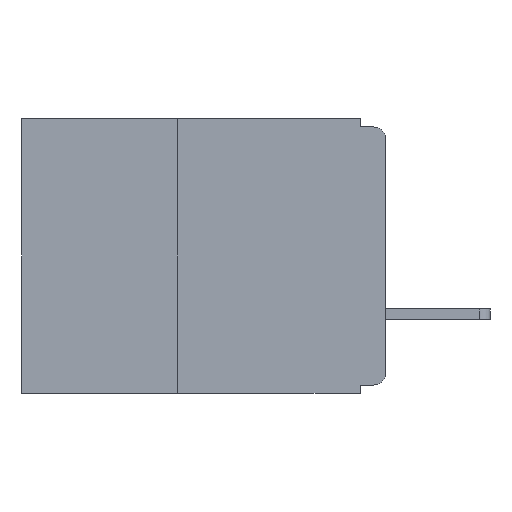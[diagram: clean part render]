
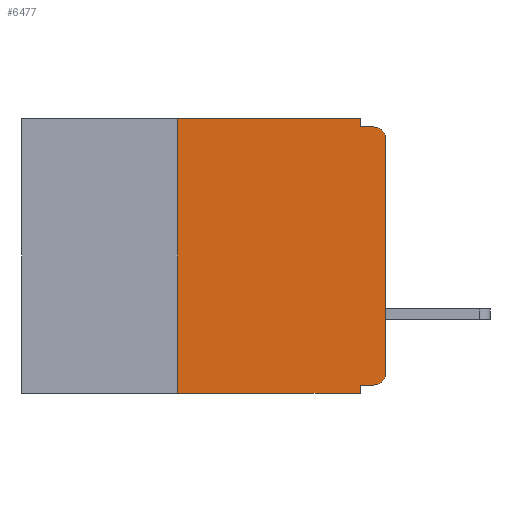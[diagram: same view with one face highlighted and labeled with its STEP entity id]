
A CAD part, left-side view. The second image highlights one B-rep face of the part: STEP entity #6477.
In plain terms, the highlighted planar face has unit normal (-1, 0, 0).
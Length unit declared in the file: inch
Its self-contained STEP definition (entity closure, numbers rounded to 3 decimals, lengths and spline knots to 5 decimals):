
#161 = ORIENTED_EDGE ( 'NONE', *, *, #11580, .F. ) ;
#552 = CARTESIAN_POINT ( 'NONE',  ( 0., 0., -0.01 ) ) ;
#624 = DIRECTION ( 'NONE',  ( 0., -1., 0. ) ) ;
#944 = VERTEX_POINT ( 'NONE', #4476 ) ;
#1103 = DIRECTION ( 'NONE',  ( -1., 0., 0. ) ) ;
#2152 = CARTESIAN_POINT ( 'NONE',  ( 0., 0.031, -0.33 ) ) ;
#2532 = EDGE_CURVE ( 'NONE', #5819, #17092, #18656, .T. ) ;
#2851 = DIRECTION ( 'NONE',  ( 0., 0., 1. ) ) ;
#3245 = VECTOR ( 'NONE', #624, 39.37008 ) ;
#3346 = CARTESIAN_POINT ( 'NONE',  ( 0., 0.25, 0. ) ) ;
#3516 = VERTEX_POINT ( 'NONE', #11714 ) ;
#3613 = LINE ( 'NONE', #552, #12341 ) ;
#3626 = ORIENTED_EDGE ( 'NONE', *, *, #19612, .T. ) ;
#3644 = CARTESIAN_POINT ( 'NONE',  ( 0., 0.031, -0.32 ) ) ;
#3839 = CARTESIAN_POINT ( 'NONE',  ( 0., 0.25, -0.33 ) ) ;
#4476 = CARTESIAN_POINT ( 'NONE',  ( 0., 0.015, -0.32 ) ) ;
#5031 = CARTESIAN_POINT ( 'NONE',  ( 0., 0.015, -0.01 ) ) ;
#5152 = ORIENTED_EDGE ( 'NONE', *, *, #12408, .T. ) ;
#5431 = CARTESIAN_POINT ( 'NONE',  ( 0., 0.031, 0. ) ) ;
#5499 = DIRECTION ( 'NONE',  ( 0., 0., -1. ) ) ;
#5501 = DIRECTION ( 'NONE',  ( 1., 0., 0. ) ) ;
#5657 = PLANE ( 'NONE',  #17679 ) ;
#5690 = LINE ( 'NONE', #8557, #14401 ) ;
#5729 = CARTESIAN_POINT ( 'NONE',  ( 0., 0.437, 0. ) ) ;
#5819 = VERTEX_POINT ( 'NONE', #21030 ) ;
#6320 = AXIS2_PLACEMENT_3D ( 'NONE', #11506, #1103, #13298 ) ;
#6477 = ADVANCED_FACE ( 'NONE', ( #7716 ), #5657, .F. ) ;
#6663 = ORIENTED_EDGE ( 'NONE', *, *, #12647, .F. ) ;
#6721 = ORIENTED_EDGE ( 'NONE', *, *, #19147, .F. ) ;
#7189 = EDGE_CURVE ( 'NONE', #19996, #3516, #12855, .T. ) ;
#7716 = FACE_OUTER_BOUND ( 'NONE', #10696, .T. ) ;
#7891 = LINE ( 'NONE', #11055, #3245 ) ;
#8170 = VERTEX_POINT ( 'NONE', #2152 ) ;
#8555 = VERTEX_POINT ( 'NONE', #5031 ) ;
#8557 = CARTESIAN_POINT ( 'NONE',  ( 0., 0., -0.32 ) ) ;
#8619 = CARTESIAN_POINT ( 'NONE',  ( 0., 0.031, -0.33 ) ) ;
#8754 = CIRCLE ( 'NONE', #19725, 0.015 ) ;
#9518 = CARTESIAN_POINT ( 'NONE',  ( 0., 0.015, -0.025 ) ) ;
#10535 = CARTESIAN_POINT ( 'NONE',  ( 0., 0.031, -0.01 ) ) ;
#10696 = EDGE_LOOP ( 'NONE', ( #18033, #5152, #161, #20203, #15067, #21837, #20244, #6663, #6721, #3626 ) ) ;
#11055 = CARTESIAN_POINT ( 'NONE',  ( 0., 0.437, -0.33 ) ) ;
#11281 = DIRECTION ( 'NONE',  ( 0., 0., -1. ) ) ;
#11506 = CARTESIAN_POINT ( 'NONE',  ( 0., 0.015, -0.305 ) ) ;
#11580 = EDGE_CURVE ( 'NONE', #13933, #8555, #3613, .T. ) ;
#11679 = DIRECTION ( 'NONE',  ( 0., 0., 1. ) ) ;
#11714 = CARTESIAN_POINT ( 'NONE',  ( 0., 0., -0.025 ) ) ;
#12341 = VECTOR ( 'NONE', #12736, 39.37008 ) ;
#12408 = EDGE_CURVE ( 'NONE', #3516, #8555, #8754, .T. ) ;
#12574 = CARTESIAN_POINT ( 'NONE',  ( 0., 0., -0.305 ) ) ;
#12647 = EDGE_CURVE ( 'NONE', #18628, #8170, #17695, .T. ) ;
#12736 = DIRECTION ( 'NONE',  ( 0., -1., 0. ) ) ;
#12855 = LINE ( 'NONE', #21897, #21871 ) ;
#13130 = VECTOR ( 'NONE', #20693, 39.37008 ) ;
#13298 = DIRECTION ( 'NONE',  ( 0., 0., -1. ) ) ;
#13933 = VERTEX_POINT ( 'NONE', #10535 ) ;
#14125 = VECTOR ( 'NONE', #2851, 39.37008 ) ;
#14271 = LINE ( 'NONE', #17498, #18278 ) ;
#14401 = VECTOR ( 'NONE', #20570, 39.37008 ) ;
#14934 = CIRCLE ( 'NONE', #6320, 0.015 ) ;
#15067 = ORIENTED_EDGE ( 'NONE', *, *, #22327, .F. ) ;
#15164 = VECTOR ( 'NONE', #21549, 39.37008 ) ;
#15699 = LINE ( 'NONE', #19882, #15164 ) ;
#17092 = VERTEX_POINT ( 'NONE', #3346 ) ;
#17199 = VERTEX_POINT ( 'NONE', #5431 ) ;
#17498 = CARTESIAN_POINT ( 'NONE',  ( 0., 0.437, 0. ) ) ;
#17679 = AXIS2_PLACEMENT_3D ( 'NONE', #5729, #5501, #5499 ) ;
#17695 = LINE ( 'NONE', #8619, #13130 ) ;
#18033 = ORIENTED_EDGE ( 'NONE', *, *, #7189, .T. ) ;
#18246 = EDGE_CURVE ( 'NONE', #5819, #8170, #7891, .T. ) ;
#18278 = VECTOR ( 'NONE', #19166, 39.37008 ) ;
#18628 = VERTEX_POINT ( 'NONE', #3644 ) ;
#18656 = LINE ( 'NONE', #3839, #14125 ) ;
#19147 = EDGE_CURVE ( 'NONE', #944, #18628, #5690, .T. ) ;
#19166 = DIRECTION ( 'NONE',  ( 0., -1., 0. ) ) ;
#19612 = EDGE_CURVE ( 'NONE', #944, #19996, #14934, .T. ) ;
#19725 = AXIS2_PLACEMENT_3D ( 'NONE', #9518, #21494, #11281 ) ;
#19882 = CARTESIAN_POINT ( 'NONE',  ( 0., 0.031, 0. ) ) ;
#19996 = VERTEX_POINT ( 'NONE', #12574 ) ;
#20154 = EDGE_CURVE ( 'NONE', #17199, #13933, #15699, .T. ) ;
#20203 = ORIENTED_EDGE ( 'NONE', *, *, #20154, .F. ) ;
#20244 = ORIENTED_EDGE ( 'NONE', *, *, #18246, .T. ) ;
#20570 = DIRECTION ( 'NONE',  ( 0., 1., 0. ) ) ;
#20693 = DIRECTION ( 'NONE',  ( 0., 0., -1. ) ) ;
#21030 = CARTESIAN_POINT ( 'NONE',  ( 0., 0.25, -0.33 ) ) ;
#21494 = DIRECTION ( 'NONE',  ( -1., 0., 0. ) ) ;
#21549 = DIRECTION ( 'NONE',  ( 0., 0., -1. ) ) ;
#21837 = ORIENTED_EDGE ( 'NONE', *, *, #2532, .F. ) ;
#21871 = VECTOR ( 'NONE', #11679, 39.37008 ) ;
#21897 = CARTESIAN_POINT ( 'NONE',  ( 0., 0., 0. ) ) ;
#22327 = EDGE_CURVE ( 'NONE', #17092, #17199, #14271, .T. ) ;
